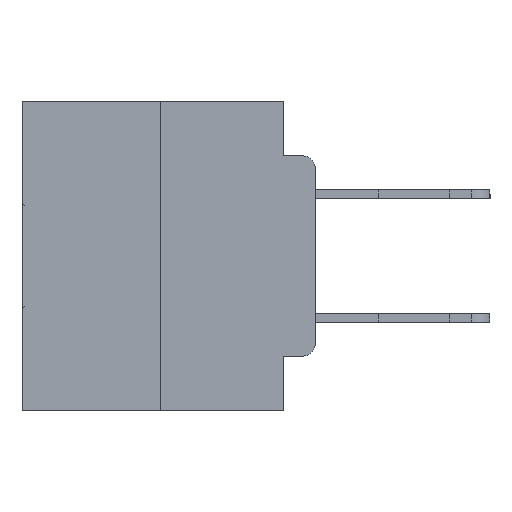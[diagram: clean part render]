
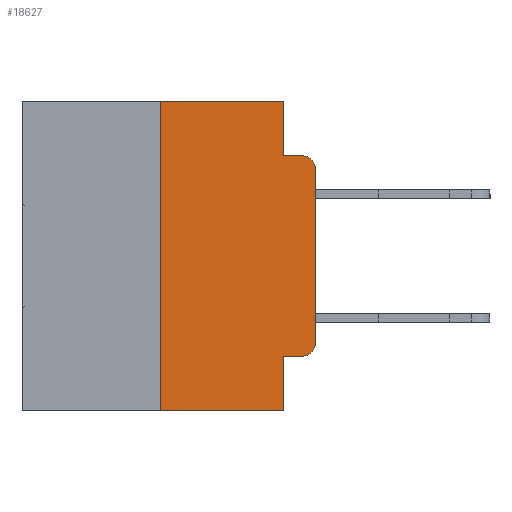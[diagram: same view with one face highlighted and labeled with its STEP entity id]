
A CAD part, left-side view. The second image highlights one B-rep face of the part: STEP entity #18627.
In plain terms, the highlighted planar face has unit normal (-1, 0, 0).
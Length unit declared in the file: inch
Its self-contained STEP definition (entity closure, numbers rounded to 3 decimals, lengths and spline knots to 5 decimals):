
#641 = VECTOR ( 'NONE', #4427, 39.37008 ) ;
#966 = VECTOR ( 'NONE', #13005, 39.37008 ) ;
#1018 = ORIENTED_EDGE ( 'NONE', *, *, #28693, .T. ) ;
#1269 = VERTEX_POINT ( 'NONE', #3527 ) ;
#2164 = LINE ( 'NONE', #19733, #19780 ) ;
#2531 = ORIENTED_EDGE ( 'NONE', *, *, #19162, .F. ) ;
#2778 = CARTESIAN_POINT ( 'NONE',  ( 0., 0.02, -0.1085 ) ) ;
#3072 = VECTOR ( 'NONE', #23126, 39.37008 ) ;
#3101 = ORIENTED_EDGE ( 'NONE', *, *, #6486, .T. ) ;
#3527 = CARTESIAN_POINT ( 'NONE',  ( 0., 0.25, -0.5 ) ) ;
#3612 = EDGE_CURVE ( 'NONE', #24716, #18111, #11518, .T. ) ;
#3621 = CARTESIAN_POINT ( 'NONE',  ( 0., 0.02, -0.4115 ) ) ;
#3637 = DIRECTION ( 'NONE',  ( 0., 0., 1. ) ) ;
#3850 = ORIENTED_EDGE ( 'NONE', *, *, #3612, .T. ) ;
#4049 = DIRECTION ( 'NONE',  ( 0., 0., -1. ) ) ;
#4427 = DIRECTION ( 'NONE',  ( 0., -1., 0. ) ) ;
#4431 = CARTESIAN_POINT ( 'NONE',  ( 0., 0., -0.1085 ) ) ;
#5070 = DIRECTION ( 'NONE',  ( 0., 0., -1. ) ) ;
#5690 = CARTESIAN_POINT ( 'NONE',  ( 0., 0.051, -0.4115 ) ) ;
#5694 = EDGE_CURVE ( 'NONE', #27162, #6246, #16128, .T. ) ;
#6022 = CARTESIAN_POINT ( 'NONE',  ( 0., 0.051, -0.4115 ) ) ;
#6228 = DIRECTION ( 'NONE',  ( 0., -1., 0. ) ) ;
#6246 = VERTEX_POINT ( 'NONE', #21940 ) ;
#6286 = CARTESIAN_POINT ( 'NONE',  ( 0., 0.051, 0. ) ) ;
#6486 = EDGE_CURVE ( 'NONE', #1269, #22984, #25050, .T. ) ;
#6522 = CARTESIAN_POINT ( 'NONE',  ( 0., 0.051, -0.5 ) ) ;
#7631 = DIRECTION ( 'NONE',  ( 0., 0., 1. ) ) ;
#7643 = CARTESIAN_POINT ( 'NONE',  ( 0., 0.051, 0. ) ) ;
#7800 = CARTESIAN_POINT ( 'NONE',  ( 0., 0.473, 0. ) ) ;
#7820 = ORIENTED_EDGE ( 'NONE', *, *, #9743, .T. ) ;
#7967 = LINE ( 'NONE', #21415, #20242 ) ;
#8425 = LINE ( 'NONE', #20173, #9155 ) ;
#8874 = CARTESIAN_POINT ( 'NONE',  ( 0., 0.02, -0.3915 ) ) ;
#9043 = AXIS2_PLACEMENT_3D ( 'NONE', #8874, #24937, #11187 ) ;
#9155 = VECTOR ( 'NONE', #4049, 39.37008 ) ;
#9247 = ORIENTED_EDGE ( 'NONE', *, *, #18792, .F. ) ;
#9352 = CARTESIAN_POINT ( 'NONE',  ( 0., 0.473, 0. ) ) ;
#9490 = VERTEX_POINT ( 'NONE', #4431 ) ;
#9743 = EDGE_CURVE ( 'NONE', #11322, #9490, #7967, .T. ) ;
#9881 = LINE ( 'NONE', #9352, #3072 ) ;
#10126 = DIRECTION ( 'NONE',  ( 1., 0., 0. ) ) ;
#10640 = FACE_OUTER_BOUND ( 'NONE', #25385, .T. ) ;
#10697 = CARTESIAN_POINT ( 'NONE',  ( 0., 0.051, -0.0885 ) ) ;
#10804 = VECTOR ( 'NONE', #6228, 39.37008 ) ;
#11187 = DIRECTION ( 'NONE',  ( 0., 0., -1. ) ) ;
#11322 = VERTEX_POINT ( 'NONE', #15527 ) ;
#11518 = LINE ( 'NONE', #6022, #10804 ) ;
#13005 = DIRECTION ( 'NONE',  ( 0., -1., 0. ) ) ;
#13523 = ORIENTED_EDGE ( 'NONE', *, *, #21045, .T. ) ;
#13663 = CIRCLE ( 'NONE', #9043, 0.02 ) ;
#14415 = EDGE_CURVE ( 'NONE', #22203, #27162, #9881, .T. ) ;
#15527 = CARTESIAN_POINT ( 'NONE',  ( 0., 0., -0.3915 ) ) ;
#16128 = LINE ( 'NONE', #6286, #27564 ) ;
#16855 = CIRCLE ( 'NONE', #26460, 0.02 ) ;
#18111 = VERTEX_POINT ( 'NONE', #3621 ) ;
#18214 = CARTESIAN_POINT ( 'NONE',  ( 0., 0.02, -0.0885 ) ) ;
#18627 = ADVANCED_FACE ( 'NONE', ( #10640 ), #23871, .F. ) ;
#18792 = EDGE_CURVE ( 'NONE', #6246, #29139, #19307, .T. ) ;
#18849 = DIRECTION ( 'NONE',  ( -1., 0., 0. ) ) ;
#18951 = ORIENTED_EDGE ( 'NONE', *, *, #5694, .F. ) ;
#19162 = EDGE_CURVE ( 'NONE', #24716, #22984, #8425, .T. ) ;
#19307 = LINE ( 'NONE', #10697, #966 ) ;
#19733 = CARTESIAN_POINT ( 'NONE',  ( 0., 0.25, 0. ) ) ;
#19780 = VECTOR ( 'NONE', #3637, 39.37008 ) ;
#20173 = CARTESIAN_POINT ( 'NONE',  ( 0., 0.051, 0. ) ) ;
#20242 = VECTOR ( 'NONE', #7631, 39.37008 ) ;
#21045 = EDGE_CURVE ( 'NONE', #18111, #11322, #13663, .T. ) ;
#21415 = CARTESIAN_POINT ( 'NONE',  ( 0., 0., 0. ) ) ;
#21493 = EDGE_CURVE ( 'NONE', #1269, #22203, #2164, .T. ) ;
#21940 = CARTESIAN_POINT ( 'NONE',  ( 0., 0.051, -0.0885 ) ) ;
#22203 = VERTEX_POINT ( 'NONE', #23994 ) ;
#22361 = DIRECTION ( 'NONE',  ( 0., 0., -1. ) ) ;
#22984 = VERTEX_POINT ( 'NONE', #6522 ) ;
#23126 = DIRECTION ( 'NONE',  ( 0., -1., 0. ) ) ;
#23603 = ORIENTED_EDGE ( 'NONE', *, *, #14415, .F. ) ;
#23871 = PLANE ( 'NONE',  #24658 ) ;
#23994 = CARTESIAN_POINT ( 'NONE',  ( 0., 0.25, 0. ) ) ;
#24658 = AXIS2_PLACEMENT_3D ( 'NONE', #7800, #10126, #26147 ) ;
#24716 = VERTEX_POINT ( 'NONE', #5690 ) ;
#24937 = DIRECTION ( 'NONE',  ( -1., 0., 0. ) ) ;
#25050 = LINE ( 'NONE', #29526, #641 ) ;
#25385 = EDGE_LOOP ( 'NONE', ( #7820, #1018, #9247, #18951, #23603, #27536, #3101, #2531, #3850, #13523 ) ) ;
#26147 = DIRECTION ( 'NONE',  ( 0., 0., -1. ) ) ;
#26460 = AXIS2_PLACEMENT_3D ( 'NONE', #2778, #18849, #5070 ) ;
#27162 = VERTEX_POINT ( 'NONE', #7643 ) ;
#27536 = ORIENTED_EDGE ( 'NONE', *, *, #21493, .F. ) ;
#27564 = VECTOR ( 'NONE', #22361, 39.37008 ) ;
#28693 = EDGE_CURVE ( 'NONE', #9490, #29139, #16855, .T. ) ;
#29139 = VERTEX_POINT ( 'NONE', #18214 ) ;
#29526 = CARTESIAN_POINT ( 'NONE',  ( 0., 0.473, -0.5 ) ) ;
